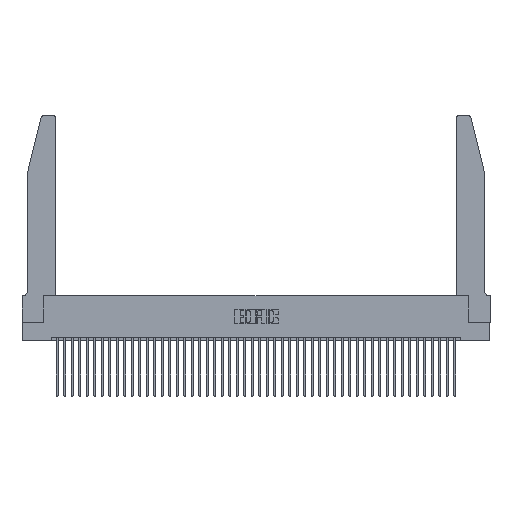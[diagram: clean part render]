
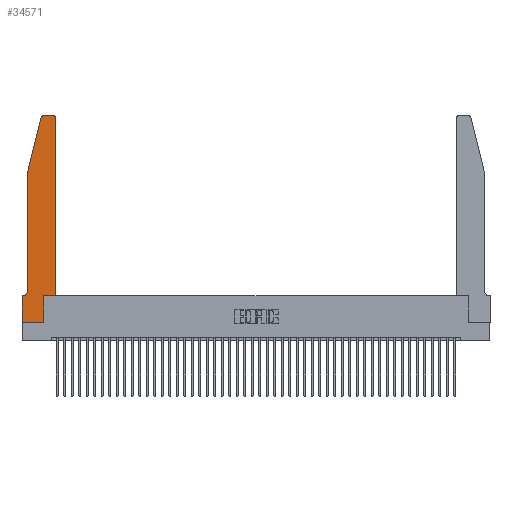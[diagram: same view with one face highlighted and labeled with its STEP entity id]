
A CAD part, top view. The second image highlights one B-rep face of the part: STEP entity #34571.
In plain terms, the highlighted planar face has unit normal (0, 0, 1).
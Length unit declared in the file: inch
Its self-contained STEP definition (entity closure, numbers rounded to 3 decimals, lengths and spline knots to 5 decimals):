
#78 = EDGE_CURVE ( 'NONE', #21668, #38367, #38511, .T. ) ;
#599 = DIRECTION ( 'NONE',  ( 0., 0., -1. ) ) ;
#765 = LINE ( 'NONE', #3205, #45328 ) ;
#1566 = DIRECTION ( 'NONE',  ( -1., 0., 0. ) ) ;
#2424 = VERTEX_POINT ( 'NONE', #23542 ) ;
#3205 = CARTESIAN_POINT ( 'NONE',  ( 0.0755, 0.35, 0.37 ) ) ;
#3401 = CARTESIAN_POINT ( 'NONE',  ( 0.2865, 0., 0.37 ) ) ;
#3707 = CARTESIAN_POINT ( 'NONE',  ( 0.0755, 2., 0.37 ) ) ;
#4260 = ORIENTED_EDGE ( 'NONE', *, *, #16406, .T. ) ;
#4685 = CARTESIAN_POINT ( 'NONE',  ( 0.2865, 0.35, 0.37 ) ) ;
#5101 = EDGE_CURVE ( 'NONE', #28429, #2424, #42485, .T. ) ;
#5174 = VECTOR ( 'NONE', #25894, 39.37008 ) ;
#5431 = CARTESIAN_POINT ( 'NONE',  ( 0.0755, 2., 0.37 ) ) ;
#8060 = EDGE_CURVE ( 'NONE', #22063, #17338, #36356, .T. ) ;
#8246 = ORIENTED_EDGE ( 'NONE', *, *, #11535, .T. ) ;
#8299 = VECTOR ( 'NONE', #37800, 39.37008 ) ;
#8431 = ORIENTED_EDGE ( 'NONE', *, *, #26626, .T. ) ;
#8688 = CARTESIAN_POINT ( 'NONE',  ( 0.4205, 2.72, 0.37 ) ) ;
#9029 = DIRECTION ( 'NONE',  ( -0.239, -0.971, 0. ) ) ;
#9354 = ORIENTED_EDGE ( 'NONE', *, *, #40144, .T. ) ;
#9547 = DIRECTION ( 'NONE',  ( 0., 0., 1. ) ) ;
#9925 = VECTOR ( 'NONE', #31408, 39.37008 ) ;
#11184 = CARTESIAN_POINT ( 'NONE',  ( 0.0755, 0.42, 0.37 ) ) ;
#11535 = EDGE_CURVE ( 'NONE', #29411, #21668, #43137, .T. ) ;
#11838 = CARTESIAN_POINT ( 'NONE',  ( 0.4505, 2.72, 0.37 ) ) ;
#12297 = DIRECTION ( 'NONE',  ( 1., 0., 0. ) ) ;
#16161 = VERTEX_POINT ( 'NONE', #25990 ) ;
#16290 = ORIENTED_EDGE ( 'NONE', *, *, #32034, .T. ) ;
#16406 = EDGE_CURVE ( 'NONE', #36662, #16161, #765, .T. ) ;
#17041 = DIRECTION ( 'NONE',  ( 0., 0., 1. ) ) ;
#17338 = VERTEX_POINT ( 'NONE', #11184 ) ;
#17606 = LINE ( 'NONE', #40975, #26903 ) ;
#17820 = VECTOR ( 'NONE', #42384, 39.37008 ) ;
#18194 = AXIS2_PLACEMENT_3D ( 'NONE', #8688, #33264, #12297 ) ;
#19735 = VERTEX_POINT ( 'NONE', #34623 ) ;
#20068 = LINE ( 'NONE', #5431, #37484 ) ;
#21235 = EDGE_CURVE ( 'NONE', #17338, #36662, #42777, .T. ) ;
#21292 = CARTESIAN_POINT ( 'NONE',  ( 0.4505, 0.35, 0.37 ) ) ;
#21668 = VERTEX_POINT ( 'NONE', #38055 ) ;
#21736 = ORIENTED_EDGE ( 'NONE', *, *, #5101, .T. ) ;
#21740 = CARTESIAN_POINT ( 'NONE',  ( 0.25487, 2.72718, 0.37 ) ) ;
#21844 = VERTEX_POINT ( 'NONE', #38795 ) ;
#21959 = CARTESIAN_POINT ( 'NONE',  ( 0.0055, 0.42, 0.37 ) ) ;
#22063 = VERTEX_POINT ( 'NONE', #29832 ) ;
#22797 = CARTESIAN_POINT ( 'NONE',  ( 0.284, 2.75, 0.37 ) ) ;
#23542 = CARTESIAN_POINT ( 'NONE',  ( 0.2865, 0.35, 0.37 ) ) ;
#23922 = PLANE ( 'NONE',  #41097 ) ;
#24178 = ORIENTED_EDGE ( 'NONE', *, *, #43858, .T. ) ;
#25481 = DIRECTION ( 'NONE',  ( -1., 0., 0. ) ) ;
#25894 = DIRECTION ( 'NONE',  ( 0., 1., 0. ) ) ;
#25990 = CARTESIAN_POINT ( 'NONE',  ( 0., 0.35, 0.37 ) ) ;
#26626 = EDGE_CURVE ( 'NONE', #16161, #19735, #17606, .T. ) ;
#26691 = CIRCLE ( 'NONE', #45150, 0.03 ) ;
#26903 = VECTOR ( 'NONE', #42210, 39.37008 ) ;
#27923 = CARTESIAN_POINT ( 'NONE',  ( 0.4505, 0.35, 0.37 ) ) ;
#28185 = LINE ( 'NONE', #34304, #8299 ) ;
#28355 = AXIS2_PLACEMENT_3D ( 'NONE', #21959, #599, #25481 ) ;
#28429 = VERTEX_POINT ( 'NONE', #3401 ) ;
#28680 = LINE ( 'NONE', #27923, #9925 ) ;
#29288 = VECTOR ( 'NONE', #1566, 39.37008 ) ;
#29411 = VERTEX_POINT ( 'NONE', #11838 ) ;
#29832 = CARTESIAN_POINT ( 'NONE',  ( 0.0755, 2., 0.37 ) ) ;
#30616 = CARTESIAN_POINT ( 'NONE',  ( 0.284, 2.72, 0.37 ) ) ;
#30766 = EDGE_CURVE ( 'NONE', #38367, #38168, #26691, .T. ) ;
#31408 = DIRECTION ( 'NONE',  ( 0., 1., 0. ) ) ;
#31459 = DIRECTION ( 'NONE',  ( -1., 0., 0. ) ) ;
#31650 = EDGE_LOOP ( 'NONE', ( #35808, #39493, #9354, #41068, #42473, #4260, #8431, #16290, #21736, #33165, #24178, #8246 ) ) ;
#31798 = DIRECTION ( 'NONE',  ( 1., 0., 0. ) ) ;
#32034 = EDGE_CURVE ( 'NONE', #19735, #28429, #28185, .T. ) ;
#33165 = ORIENTED_EDGE ( 'NONE', *, *, #37105, .T. ) ;
#33235 = CARTESIAN_POINT ( 'NONE',  ( 0.2605, 2.75, 0.37 ) ) ;
#33264 = DIRECTION ( 'NONE',  ( 0., 0., 1. ) ) ;
#33414 = VECTOR ( 'NONE', #31798, 39.37008 ) ;
#34096 = DIRECTION ( 'NONE',  ( 1., 0., 0. ) ) ;
#34304 = CARTESIAN_POINT ( 'NONE',  ( 0., 0., 0.37 ) ) ;
#34511 = LINE ( 'NONE', #21292, #33414 ) ;
#34571 = ADVANCED_FACE ( 'NONE', ( #37716 ), #23922, .T. ) ;
#34623 = CARTESIAN_POINT ( 'NONE',  ( 0., 0., 0.37 ) ) ;
#35808 = ORIENTED_EDGE ( 'NONE', *, *, #78, .T. ) ;
#36356 = LINE ( 'NONE', #3707, #17820 ) ;
#36398 = CARTESIAN_POINT ( 'NONE',  ( 0.0055, 0.35, 0.37 ) ) ;
#36662 = VERTEX_POINT ( 'NONE', #36398 ) ;
#37105 = EDGE_CURVE ( 'NONE', #2424, #21844, #34511, .T. ) ;
#37484 = VECTOR ( 'NONE', #9029, 39.37008 ) ;
#37716 = FACE_OUTER_BOUND ( 'NONE', #31650, .T. ) ;
#37800 = DIRECTION ( 'NONE',  ( 1., 0., 0. ) ) ;
#37908 = CARTESIAN_POINT ( 'NONE',  ( 0., 0.35, 0.37 ) ) ;
#38055 = CARTESIAN_POINT ( 'NONE',  ( 0.4205, 2.75, 0.37 ) ) ;
#38168 = VERTEX_POINT ( 'NONE', #21740 ) ;
#38367 = VERTEX_POINT ( 'NONE', #22797 ) ;
#38511 = LINE ( 'NONE', #33235, #29288 ) ;
#38795 = CARTESIAN_POINT ( 'NONE',  ( 0.4505, 0.35, 0.37 ) ) ;
#39493 = ORIENTED_EDGE ( 'NONE', *, *, #30766, .T. ) ;
#40144 = EDGE_CURVE ( 'NONE', #38168, #22063, #20068, .T. ) ;
#40975 = CARTESIAN_POINT ( 'NONE',  ( 0., 0., 0.37 ) ) ;
#41068 = ORIENTED_EDGE ( 'NONE', *, *, #8060, .T. ) ;
#41097 = AXIS2_PLACEMENT_3D ( 'NONE', #37908, #17041, #41369 ) ;
#41369 = DIRECTION ( 'NONE',  ( 1., 0., 0. ) ) ;
#42210 = DIRECTION ( 'NONE',  ( 0., -1., 0. ) ) ;
#42384 = DIRECTION ( 'NONE',  ( 0., -1., 0. ) ) ;
#42473 = ORIENTED_EDGE ( 'NONE', *, *, #21235, .T. ) ;
#42485 = LINE ( 'NONE', #4685, #5174 ) ;
#42777 = CIRCLE ( 'NONE', #28355, 0.07 ) ;
#43137 = CIRCLE ( 'NONE', #18194, 0.03 ) ;
#43858 = EDGE_CURVE ( 'NONE', #21844, #29411, #28680, .T. ) ;
#45150 = AXIS2_PLACEMENT_3D ( 'NONE', #30616, #9547, #34096 ) ;
#45328 = VECTOR ( 'NONE', #31459, 39.37008 ) ;
